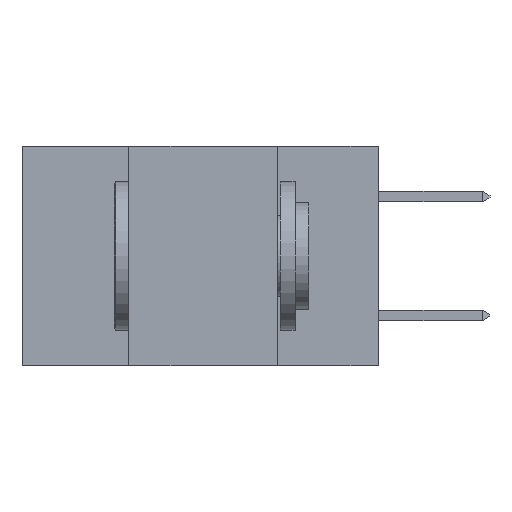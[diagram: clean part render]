
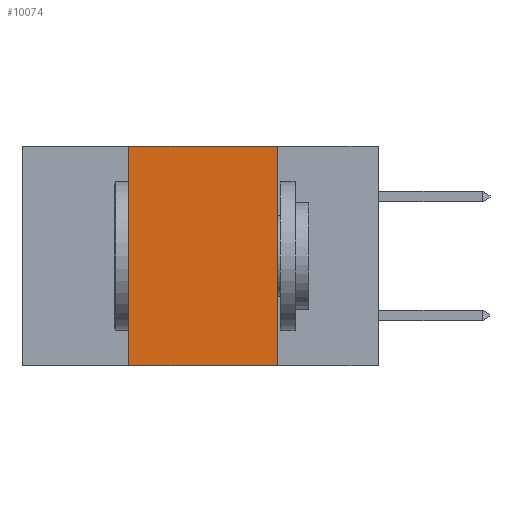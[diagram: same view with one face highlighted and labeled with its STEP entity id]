
A CAD part, left-side view. The second image highlights one B-rep face of the part: STEP entity #10074.
In plain terms, the highlighted planar face has unit normal (-1, 0, 0).
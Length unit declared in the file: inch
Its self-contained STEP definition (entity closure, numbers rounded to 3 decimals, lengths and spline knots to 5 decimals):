
#212 = EDGE_CURVE ( 'NONE', #10635, #2352, #2653, .T. ) ;
#434 = PLANE ( 'NONE',  #3672 ) ;
#448 = LINE ( 'NONE', #5216, #7615 ) ;
#1070 = VERTEX_POINT ( 'NONE', #2614 ) ;
#1470 = LINE ( 'NONE', #7354, #3817 ) ;
#1648 = ORIENTED_EDGE ( 'NONE', *, *, #2505, .T. ) ;
#1916 = VECTOR ( 'NONE', #5854, 39.37008 ) ;
#2352 = VERTEX_POINT ( 'NONE', #6429 ) ;
#2418 = EDGE_CURVE ( 'NONE', #4048, #1070, #1470, .T. ) ;
#2505 = EDGE_CURVE ( 'NONE', #10635, #1070, #448, .T. ) ;
#2594 = FACE_OUTER_BOUND ( 'NONE', #2794, .T. ) ;
#2614 = CARTESIAN_POINT ( 'NONE',  ( 0., 0.17, -0.37 ) ) ;
#2653 = LINE ( 'NONE', #6667, #12088 ) ;
#2794 = EDGE_LOOP ( 'NONE', ( #5673, #10368, #7482, #1648 ) ) ;
#3526 = DIRECTION ( 'NONE',  ( 0., 0., -1. ) ) ;
#3672 = AXIS2_PLACEMENT_3D ( 'NONE', #7296, #9061, #3526 ) ;
#3817 = VECTOR ( 'NONE', #5251, 39.37008 ) ;
#4048 = VERTEX_POINT ( 'NONE', #6314 ) ;
#4481 = LINE ( 'NONE', #10232, #1916 ) ;
#4550 = EDGE_CURVE ( 'NONE', #2352, #4048, #4481, .T. ) ;
#5216 = CARTESIAN_POINT ( 'NONE',  ( 0., 0.6, -0.37 ) ) ;
#5251 = DIRECTION ( 'NONE',  ( 0., 0., -1. ) ) ;
#5673 = ORIENTED_EDGE ( 'NONE', *, *, #2418, .F. ) ;
#5854 = DIRECTION ( 'NONE',  ( 0., -1., 0. ) ) ;
#6314 = CARTESIAN_POINT ( 'NONE',  ( 0., 0.17, 0. ) ) ;
#6429 = CARTESIAN_POINT ( 'NONE',  ( 0., 0.42, 0. ) ) ;
#6667 = CARTESIAN_POINT ( 'NONE',  ( 0., 0.42, 0. ) ) ;
#6986 = DIRECTION ( 'NONE',  ( 0., -1., 0. ) ) ;
#7014 = DIRECTION ( 'NONE',  ( 0., 0., 1. ) ) ;
#7296 = CARTESIAN_POINT ( 'NONE',  ( 0., 0.6, 0. ) ) ;
#7354 = CARTESIAN_POINT ( 'NONE',  ( 0., 0.17, 0. ) ) ;
#7482 = ORIENTED_EDGE ( 'NONE', *, *, #212, .F. ) ;
#7615 = VECTOR ( 'NONE', #6986, 39.37008 ) ;
#9061 = DIRECTION ( 'NONE',  ( 1., 0., 0. ) ) ;
#10074 = ADVANCED_FACE ( 'NONE', ( #2594 ), #434, .F. ) ;
#10232 = CARTESIAN_POINT ( 'NONE',  ( 0., 0.6, 0. ) ) ;
#10368 = ORIENTED_EDGE ( 'NONE', *, *, #4550, .F. ) ;
#10572 = CARTESIAN_POINT ( 'NONE',  ( 0., 0.42, -0.37 ) ) ;
#10635 = VERTEX_POINT ( 'NONE', #10572 ) ;
#12088 = VECTOR ( 'NONE', #7014, 39.37008 ) ;
